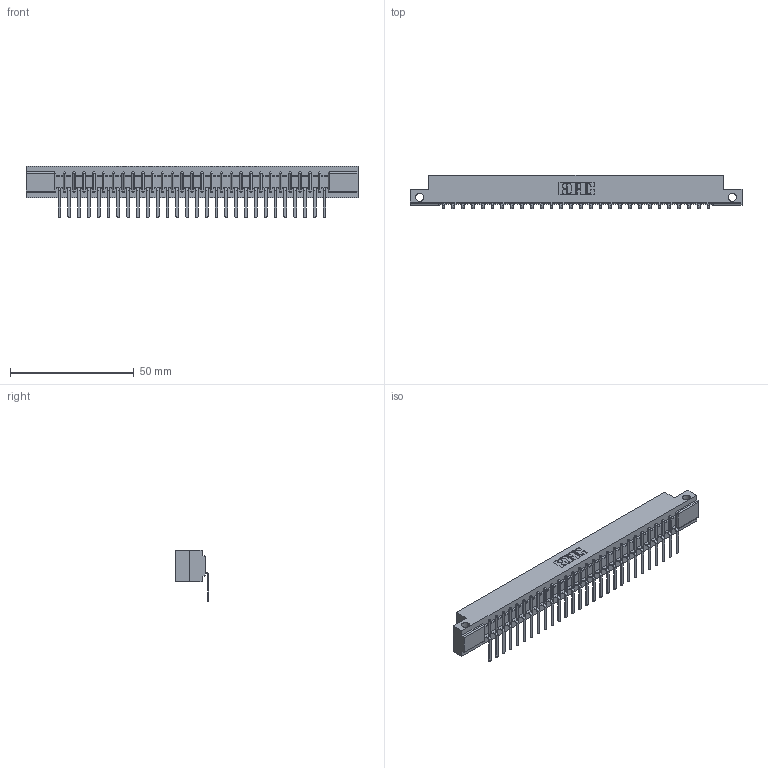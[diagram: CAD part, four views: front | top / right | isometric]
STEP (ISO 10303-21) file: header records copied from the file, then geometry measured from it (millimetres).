
FILE_DESCRIPTION (( 'STEP AP203' ), '1' );
FILE_NAME ('307-028-457-112.STEP', '2020-09-28T08:02:29', ( '' ), ( '' ), 'SwSTEP 2.0', 'SolidWorks 2020', '' );
FILE_SCHEMA (( 'CONFIG_CONTROL_DESIGN' ));
Length unit declared in the file: inch
Products named in the file (3): 307-290-002_557; 307-028-457-112; 307 Part_.128 Dia Side Mounting Holes
Assembly tree (29 placements, depth 2):
  307-028-457-112
    307 Part_.128 Dia Side Mounting Holes
    307-290-002_557  x28
Bounding box: 133.96 x 13.32 x 20.66 mm (x, y, z)
Volume: 14164.4 mm3; surface area: 17983.5 mm2
Topology: 29 solids, 29 shells, 2331 faces, 7155 edges, 4690 vertices
Faces by surface type: plane 1386, cylinder 887, sphere 58
Entity records: 26586 total; most frequent: CARTESIAN_POINT 4484, ORIENTED_EDGE 4474, DIRECTION 4363, EDGE_CURVE 2237, LINE 1705, VECTOR 1705, VERTEX_POINT 1450, AXIS2_PLACEMENT_3D 1329
